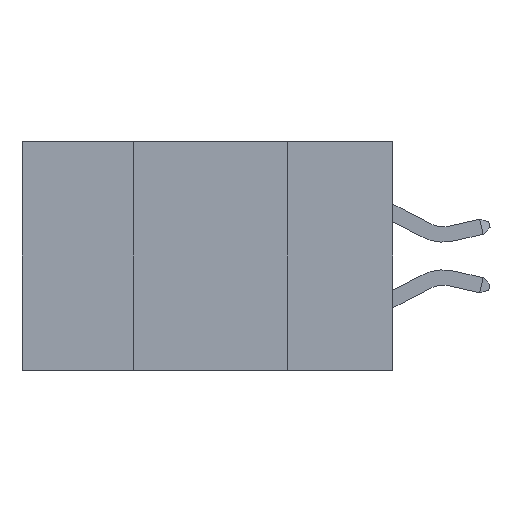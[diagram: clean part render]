
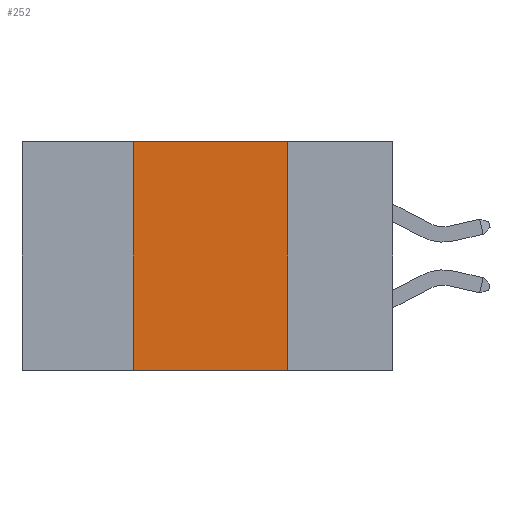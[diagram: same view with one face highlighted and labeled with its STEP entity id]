
A CAD part, left-side view. The second image highlights one B-rep face of the part: STEP entity #252.
In plain terms, the highlighted planar face has unit normal (-1, 0, 0).
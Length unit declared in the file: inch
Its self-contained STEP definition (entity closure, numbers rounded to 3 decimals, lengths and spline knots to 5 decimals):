
#252 = ADVANCED_FACE ( 'NONE', ( #5436 ), #8132, .F. ) ;
#269 = CARTESIAN_POINT ( 'NONE',  ( 0., 0.17, 0. ) ) ;
#1341 = ORIENTED_EDGE ( 'NONE', *, *, #12319, .F. ) ;
#1443 = VERTEX_POINT ( 'NONE', #269 ) ;
#1731 = ORIENTED_EDGE ( 'NONE', *, *, #5003, .T. ) ;
#2258 = DIRECTION ( 'NONE',  ( 0., 0., -1. ) ) ;
#2580 = DIRECTION ( 'NONE',  ( 1., 0., 0. ) ) ;
#3180 = VECTOR ( 'NONE', #12546, 39.37008 ) ;
#3823 = VERTEX_POINT ( 'NONE', #9680 ) ;
#4266 = ORIENTED_EDGE ( 'NONE', *, *, #5966, .F. ) ;
#4438 = CARTESIAN_POINT ( 'NONE',  ( 0., 0.17, -0.37 ) ) ;
#4527 = LINE ( 'NONE', #8015, #13247 ) ;
#4653 = ORIENTED_EDGE ( 'NONE', *, *, #10356, .F. ) ;
#4661 = EDGE_LOOP ( 'NONE', ( #4266, #1341, #4653, #1731 ) ) ;
#4701 = VECTOR ( 'NONE', #13673, 39.37008 ) ;
#5003 = EDGE_CURVE ( 'NONE', #6945, #7784, #13725, .T. ) ;
#5235 = CARTESIAN_POINT ( 'NONE',  ( 0., 0.42, -0.37 ) ) ;
#5436 = FACE_OUTER_BOUND ( 'NONE', #4661, .T. ) ;
#5966 = EDGE_CURVE ( 'NONE', #1443, #7784, #4527, .T. ) ;
#6524 = CARTESIAN_POINT ( 'NONE',  ( 0., 0.42, 0. ) ) ;
#6945 = VERTEX_POINT ( 'NONE', #5235 ) ;
#7603 = CARTESIAN_POINT ( 'NONE',  ( 0., 0.6, 0. ) ) ;
#7784 = VERTEX_POINT ( 'NONE', #4438 ) ;
#7850 = VECTOR ( 'NONE', #12189, 39.37008 ) ;
#8015 = CARTESIAN_POINT ( 'NONE',  ( 0., 0.17, 0. ) ) ;
#8132 = PLANE ( 'NONE',  #8975 ) ;
#8975 = AXIS2_PLACEMENT_3D ( 'NONE', #7603, #2580, #2258 ) ;
#9214 = DIRECTION ( 'NONE',  ( 0., 0., -1. ) ) ;
#9680 = CARTESIAN_POINT ( 'NONE',  ( 0., 0.42, 0. ) ) ;
#9951 = LINE ( 'NONE', #10409, #3180 ) ;
#10356 = EDGE_CURVE ( 'NONE', #6945, #3823, #13948, .T. ) ;
#10409 = CARTESIAN_POINT ( 'NONE',  ( 0., 0.6, 0. ) ) ;
#12189 = DIRECTION ( 'NONE',  ( 0., 0., 1. ) ) ;
#12319 = EDGE_CURVE ( 'NONE', #3823, #1443, #9951, .T. ) ;
#12546 = DIRECTION ( 'NONE',  ( 0., -1., 0. ) ) ;
#12632 = CARTESIAN_POINT ( 'NONE',  ( 0., 0.6, -0.37 ) ) ;
#13247 = VECTOR ( 'NONE', #9214, 39.37008 ) ;
#13673 = DIRECTION ( 'NONE',  ( 0., -1., 0. ) ) ;
#13725 = LINE ( 'NONE', #12632, #4701 ) ;
#13948 = LINE ( 'NONE', #6524, #7850 ) ;
